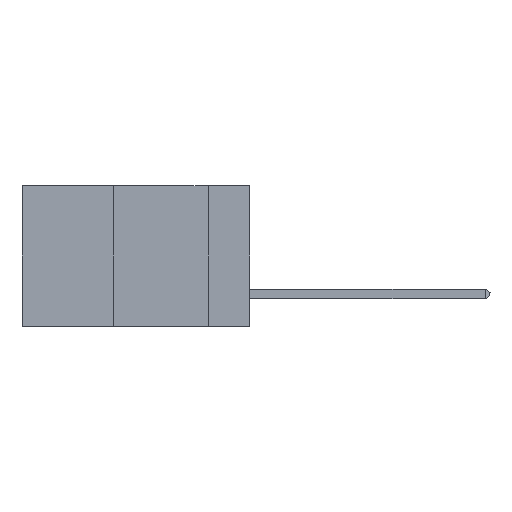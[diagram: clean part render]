
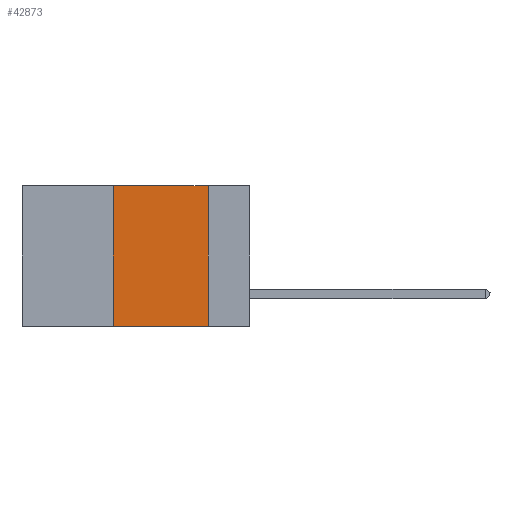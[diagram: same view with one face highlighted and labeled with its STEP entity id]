
A CAD part, left-side view. The second image highlights one B-rep face of the part: STEP entity #42873.
In plain terms, the highlighted planar face has unit normal (-1, 0, 0).
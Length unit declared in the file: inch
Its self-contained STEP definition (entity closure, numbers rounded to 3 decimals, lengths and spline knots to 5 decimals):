
#2528 = DIRECTION ( 'NONE',  ( 1., 0., 0. ) ) ;
#3354 = LINE ( 'NONE', #4866, #24082 ) ;
#4546 = DIRECTION ( 'NONE',  ( 0., -1., 0. ) ) ;
#4866 = CARTESIAN_POINT ( 'NONE',  ( 0., 0.6, -0.37 ) ) ;
#7799 = VERTEX_POINT ( 'NONE', #23467 ) ;
#7951 = VERTEX_POINT ( 'NONE', #19876 ) ;
#10071 = CARTESIAN_POINT ( 'NONE',  ( 0., 0.36, 0. ) ) ;
#10650 = FACE_OUTER_BOUND ( 'NONE', #24291, .T. ) ;
#11698 = LINE ( 'NONE', #44569, #42395 ) ;
#14650 = ORIENTED_EDGE ( 'NONE', *, *, #15815, .F. ) ;
#15815 = EDGE_CURVE ( 'NONE', #7951, #7799, #16055, .T. ) ;
#16055 = LINE ( 'NONE', #10071, #22589 ) ;
#18877 = ORIENTED_EDGE ( 'NONE', *, *, #30940, .T. ) ;
#19876 = CARTESIAN_POINT ( 'NONE',  ( 0., 0.36, -0.37 ) ) ;
#21387 = VERTEX_POINT ( 'NONE', #43552 ) ;
#22589 = VECTOR ( 'NONE', #25073, 39.37008 ) ;
#23467 = CARTESIAN_POINT ( 'NONE',  ( 0., 0.36, 0. ) ) ;
#24082 = VECTOR ( 'NONE', #4546, 39.37008 ) ;
#24291 = EDGE_LOOP ( 'NONE', ( #48740, #42408, #14650, #18877 ) ) ;
#25073 = DIRECTION ( 'NONE',  ( 0., 0., 1. ) ) ;
#25147 = EDGE_CURVE ( 'NONE', #46438, #21387, #11698, .T. ) ;
#25653 = DIRECTION ( 'NONE',  ( 0., 0., -1. ) ) ;
#26828 = VECTOR ( 'NONE', #39708, 39.37008 ) ;
#30940 = EDGE_CURVE ( 'NONE', #7951, #21387, #3354, .T. ) ;
#36930 = DIRECTION ( 'NONE',  ( 0., 0., -1. ) ) ;
#39378 = CARTESIAN_POINT ( 'NONE',  ( 0., 0.6, 0. ) ) ;
#39522 = EDGE_CURVE ( 'NONE', #7799, #46438, #40421, .T. ) ;
#39708 = DIRECTION ( 'NONE',  ( 0., -1., 0. ) ) ;
#40189 = CARTESIAN_POINT ( 'NONE',  ( 0., 0.6, 0. ) ) ;
#40421 = LINE ( 'NONE', #39378, #26828 ) ;
#42395 = VECTOR ( 'NONE', #36930, 39.37008 ) ;
#42408 = ORIENTED_EDGE ( 'NONE', *, *, #39522, .F. ) ;
#42873 = ADVANCED_FACE ( 'NONE', ( #10650 ), #44660, .F. ) ;
#43552 = CARTESIAN_POINT ( 'NONE',  ( 0., 0.11, -0.37 ) ) ;
#44569 = CARTESIAN_POINT ( 'NONE',  ( 0., 0.11, 0. ) ) ;
#44660 = PLANE ( 'NONE',  #46757 ) ;
#45457 = CARTESIAN_POINT ( 'NONE',  ( 0., 0.11, 0. ) ) ;
#46438 = VERTEX_POINT ( 'NONE', #45457 ) ;
#46757 = AXIS2_PLACEMENT_3D ( 'NONE', #40189, #2528, #25653 ) ;
#48740 = ORIENTED_EDGE ( 'NONE', *, *, #25147, .F. ) ;
